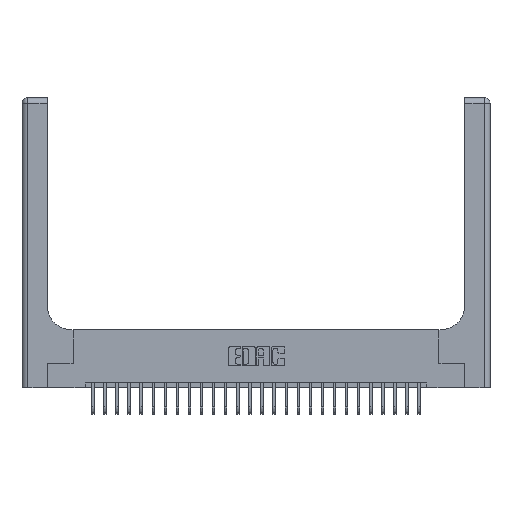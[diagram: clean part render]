
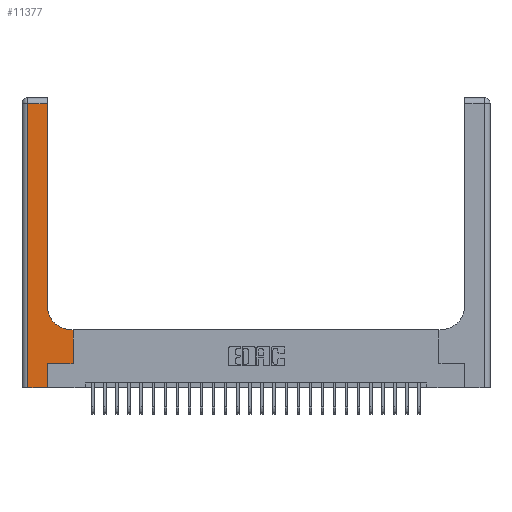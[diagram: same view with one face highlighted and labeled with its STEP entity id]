
A CAD part, top view. The second image highlights one B-rep face of the part: STEP entity #11377.
In plain terms, the highlighted planar face has unit normal (0, 0, 1).
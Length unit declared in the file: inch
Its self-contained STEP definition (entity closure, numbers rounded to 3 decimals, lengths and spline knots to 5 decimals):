
#796 = EDGE_CURVE ( 'NONE', #13424, #11008, #4705, .T. ) ;
#1039 = EDGE_CURVE ( 'NONE', #6402, #6303, #23089, .T. ) ;
#1729 = DIRECTION ( 'NONE',  ( 0., -1., 0. ) ) ;
#2233 = VERTEX_POINT ( 'NONE', #9135 ) ;
#2354 = EDGE_LOOP ( 'NONE', ( #9748, #5610, #11732, #16931, #24483, #8081, #17113, #21995, #2603 ) ) ;
#2603 = ORIENTED_EDGE ( 'NONE', *, *, #18382, .T. ) ;
#3198 = VECTOR ( 'NONE', #7959, 39.37008 ) ;
#3251 = CARTESIAN_POINT ( 'NONE',  ( 0., 3., 0.37 ) ) ;
#3521 = DIRECTION ( 'NONE',  ( -1., 0., 0. ) ) ;
#4181 = VERTEX_POINT ( 'NONE', #9334 ) ;
#4502 = CARTESIAN_POINT ( 'NONE',  ( 0.06, 0., 0.37 ) ) ;
#4688 = EDGE_CURVE ( 'NONE', #11008, #2233, #7566, .T. ) ;
#4705 = LINE ( 'NONE', #24537, #10273 ) ;
#5610 = ORIENTED_EDGE ( 'NONE', *, *, #8468, .T. ) ;
#6303 = VERTEX_POINT ( 'NONE', #20173 ) ;
#6402 = VERTEX_POINT ( 'NONE', #25099 ) ;
#7433 = LINE ( 'NONE', #27033, #3198 ) ;
#7566 = LINE ( 'NONE', #14056, #25295 ) ;
#7707 = VECTOR ( 'NONE', #3521, 39.37008 ) ;
#7959 = DIRECTION ( 'NONE',  ( 0., 1., 0. ) ) ;
#8081 = ORIENTED_EDGE ( 'NONE', *, *, #1039, .T. ) ;
#8230 = VERTEX_POINT ( 'NONE', #25454 ) ;
#8249 = EDGE_CURVE ( 'NONE', #2233, #6402, #17916, .T. ) ;
#8468 = EDGE_CURVE ( 'NONE', #22958, #13424, #13327, .T. ) ;
#9135 = CARTESIAN_POINT ( 'NONE',  ( 0.265, 0., 0.37 ) ) ;
#9190 = CIRCLE ( 'NONE', #24764, 0.25 ) ;
#9334 = CARTESIAN_POINT ( 'NONE',  ( 0.26, 0.85, 0.37 ) ) ;
#9748 = ORIENTED_EDGE ( 'NONE', *, *, #12612, .T. ) ;
#10273 = VECTOR ( 'NONE', #1729, 39.37008 ) ;
#10820 = CARTESIAN_POINT ( 'NONE',  ( 0.06, 2.94, 0.37 ) ) ;
#10891 = DIRECTION ( 'NONE',  ( 0., 1., 0. ) ) ;
#10971 = CARTESIAN_POINT ( 'NONE',  ( 0.265, 0.25, 0.37 ) ) ;
#11008 = VERTEX_POINT ( 'NONE', #4502 ) ;
#11377 = ADVANCED_FACE ( 'NONE', ( #23646 ), #11791, .F. ) ;
#11446 = LINE ( 'NONE', #25777, #22586 ) ;
#11732 = ORIENTED_EDGE ( 'NONE', *, *, #796, .T. ) ;
#11791 = PLANE ( 'NONE',  #22004 ) ;
#12612 = EDGE_CURVE ( 'NONE', #4181, #22958, #11446, .T. ) ;
#13204 = CARTESIAN_POINT ( 'NONE',  ( 0.51, 0.85, 0.37 ) ) ;
#13327 = LINE ( 'NONE', #22152, #7707 ) ;
#13424 = VERTEX_POINT ( 'NONE', #10820 ) ;
#13435 = DIRECTION ( 'NONE',  ( 0., 1., 0. ) ) ;
#14056 = CARTESIAN_POINT ( 'NONE',  ( 0., 0., 0.37 ) ) ;
#15117 = DIRECTION ( 'NONE',  ( 1., 0., 0. ) ) ;
#15132 = DIRECTION ( 'NONE',  ( 0., 0., -1. ) ) ;
#15310 = DIRECTION ( 'NONE',  ( 1., 0., 0. ) ) ;
#15577 = VECTOR ( 'NONE', #18819, 39.37008 ) ;
#15628 = VECTOR ( 'NONE', #10891, 39.37008 ) ;
#16931 = ORIENTED_EDGE ( 'NONE', *, *, #4688, .T. ) ;
#17113 = ORIENTED_EDGE ( 'NONE', *, *, #20577, .T. ) ;
#17169 = CARTESIAN_POINT ( 'NONE',  ( 0.51, 0.6, 0.37 ) ) ;
#17916 = LINE ( 'NONE', #23727, #15628 ) ;
#18382 = EDGE_CURVE ( 'NONE', #20448, #4181, #9190, .T. ) ;
#18540 = CARTESIAN_POINT ( 'NONE',  ( 0.26, 2.94, 0.37 ) ) ;
#18819 = DIRECTION ( 'NONE',  ( -1., 0., 0. ) ) ;
#19963 = DIRECTION ( 'NONE',  ( -1., 0., 0. ) ) ;
#20173 = CARTESIAN_POINT ( 'NONE',  ( 0.528, 0.25, 0.37 ) ) ;
#20374 = DIRECTION ( 'NONE',  ( 1., 0., 0. ) ) ;
#20448 = VERTEX_POINT ( 'NONE', #17169 ) ;
#20577 = EDGE_CURVE ( 'NONE', #6303, #8230, #7433, .T. ) ;
#21995 = ORIENTED_EDGE ( 'NONE', *, *, #22907, .T. ) ;
#22004 = AXIS2_PLACEMENT_3D ( 'NONE', #3251, #26445, #19963 ) ;
#22152 = CARTESIAN_POINT ( 'NONE',  ( 0., 2.94, 0.37 ) ) ;
#22586 = VECTOR ( 'NONE', #13435, 39.37008 ) ;
#22907 = EDGE_CURVE ( 'NONE', #8230, #20448, #26715, .T. ) ;
#22958 = VERTEX_POINT ( 'NONE', #18540 ) ;
#23089 = LINE ( 'NONE', #10971, #24374 ) ;
#23646 = FACE_OUTER_BOUND ( 'NONE', #2354, .T. ) ;
#23727 = CARTESIAN_POINT ( 'NONE',  ( 0.265, 0., 0.37 ) ) ;
#24374 = VECTOR ( 'NONE', #15117, 39.37008 ) ;
#24483 = ORIENTED_EDGE ( 'NONE', *, *, #8249, .T. ) ;
#24537 = CARTESIAN_POINT ( 'NONE',  ( 0.06, 3., 0.37 ) ) ;
#24764 = AXIS2_PLACEMENT_3D ( 'NONE', #13204, #15132, #15310 ) ;
#25099 = CARTESIAN_POINT ( 'NONE',  ( 0.265, 0.25, 0.37 ) ) ;
#25295 = VECTOR ( 'NONE', #20374, 39.37008 ) ;
#25454 = CARTESIAN_POINT ( 'NONE',  ( 0.528, 0.6, 0.37 ) ) ;
#25777 = CARTESIAN_POINT ( 'NONE',  ( 0.26, 3., 0.37 ) ) ;
#26445 = DIRECTION ( 'NONE',  ( 0., 0., -1. ) ) ;
#26715 = LINE ( 'NONE', #27152, #15577 ) ;
#27033 = CARTESIAN_POINT ( 'NONE',  ( 0.528, 0.25, 0.37 ) ) ;
#27152 = CARTESIAN_POINT ( 'NONE',  ( 0.26, 0.6, 0.37 ) ) ;
